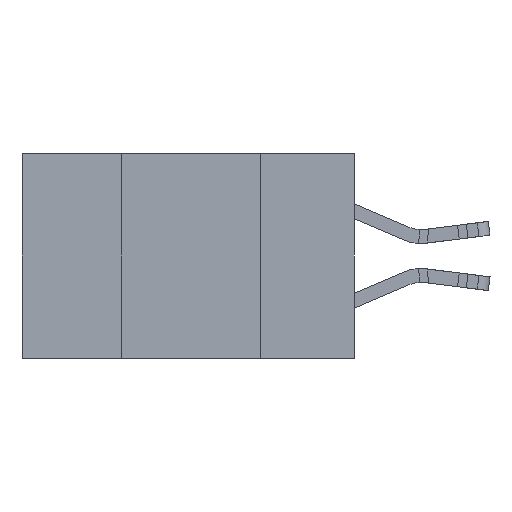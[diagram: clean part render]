
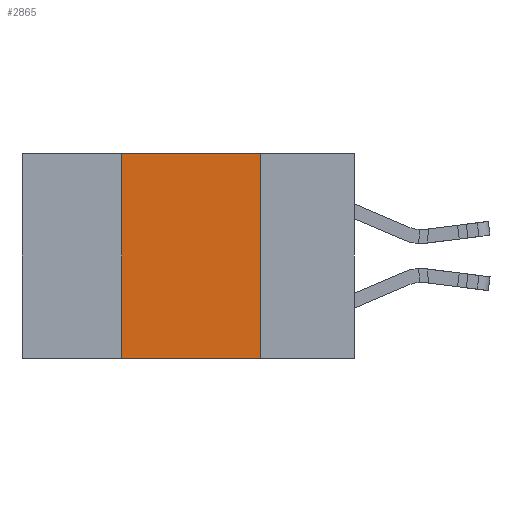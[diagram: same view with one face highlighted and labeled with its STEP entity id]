
A CAD part, left-side view. The second image highlights one B-rep face of the part: STEP entity #2865.
In plain terms, the highlighted planar face has unit normal (-1, 0, 0).
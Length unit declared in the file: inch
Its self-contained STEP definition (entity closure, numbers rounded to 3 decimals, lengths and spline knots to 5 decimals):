
#90 = VECTOR ( 'NONE', #22424, 39.37008 ) ;
#1014 = VECTOR ( 'NONE', #22607, 39.37008 ) ;
#1685 = CARTESIAN_POINT ( 'NONE',  ( 0., 0.17, -0.37 ) ) ;
#2241 = EDGE_CURVE ( 'NONE', #18417, #18511, #4963, .T. ) ;
#2827 = ORIENTED_EDGE ( 'NONE', *, *, #18401, .F. ) ;
#2865 = ADVANCED_FACE ( 'NONE', ( #21752 ), #4343, .F. ) ;
#3455 = LINE ( 'NONE', #15923, #22606 ) ;
#3476 = EDGE_CURVE ( 'NONE', #10180, #9156, #3455, .T. ) ;
#4059 = DIRECTION ( 'NONE',  ( 0., 0., -1. ) ) ;
#4093 = DIRECTION ( 'NONE',  ( 1., 0., 0. ) ) ;
#4343 = PLANE ( 'NONE',  #8223 ) ;
#4363 = CARTESIAN_POINT ( 'NONE',  ( 0., 0.6, 0. ) ) ;
#4963 = LINE ( 'NONE', #22841, #90 ) ;
#5908 = LINE ( 'NONE', #9624, #1014 ) ;
#6139 = VECTOR ( 'NONE', #21620, 39.37008 ) ;
#6711 = LINE ( 'NONE', #8726, #6139 ) ;
#7183 = EDGE_CURVE ( 'NONE', #18417, #10180, #5908, .T. ) ;
#7410 = CARTESIAN_POINT ( 'NONE',  ( 0., 0.17, 0. ) ) ;
#8223 = AXIS2_PLACEMENT_3D ( 'NONE', #4363, #4093, #4059 ) ;
#8726 = CARTESIAN_POINT ( 'NONE',  ( 0., 0.17, -0.37 ) ) ;
#9156 = VERTEX_POINT ( 'NONE', #7410 ) ;
#9494 = ORIENTED_EDGE ( 'NONE', *, *, #2241, .T. ) ;
#9624 = CARTESIAN_POINT ( 'NONE',  ( 0., 0.42, -0.37 ) ) ;
#10180 = VERTEX_POINT ( 'NONE', #16107 ) ;
#10600 = CARTESIAN_POINT ( 'NONE',  ( 0., 0.42, -0.37 ) ) ;
#14121 = EDGE_LOOP ( 'NONE', ( #2827, #23120, #18209, #9494 ) ) ;
#15092 = DIRECTION ( 'NONE',  ( 0., -1., 0. ) ) ;
#15923 = CARTESIAN_POINT ( 'NONE',  ( 0., 0.6, 0. ) ) ;
#16107 = CARTESIAN_POINT ( 'NONE',  ( 0., 0.42, 0. ) ) ;
#18209 = ORIENTED_EDGE ( 'NONE', *, *, #7183, .F. ) ;
#18401 = EDGE_CURVE ( 'NONE', #9156, #18511, #6711, .T. ) ;
#18417 = VERTEX_POINT ( 'NONE', #10600 ) ;
#18511 = VERTEX_POINT ( 'NONE', #1685 ) ;
#21620 = DIRECTION ( 'NONE',  ( 0., 0., -1. ) ) ;
#21752 = FACE_OUTER_BOUND ( 'NONE', #14121, .T. ) ;
#22424 = DIRECTION ( 'NONE',  ( 0., -1., 0. ) ) ;
#22606 = VECTOR ( 'NONE', #15092, 39.37008 ) ;
#22607 = DIRECTION ( 'NONE',  ( 0., 0., 1. ) ) ;
#22841 = CARTESIAN_POINT ( 'NONE',  ( 0., 0.6, -0.37 ) ) ;
#23120 = ORIENTED_EDGE ( 'NONE', *, *, #3476, .F. ) ;
